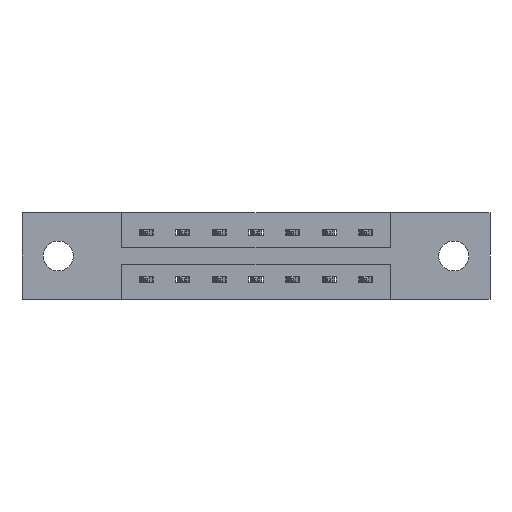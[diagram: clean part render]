
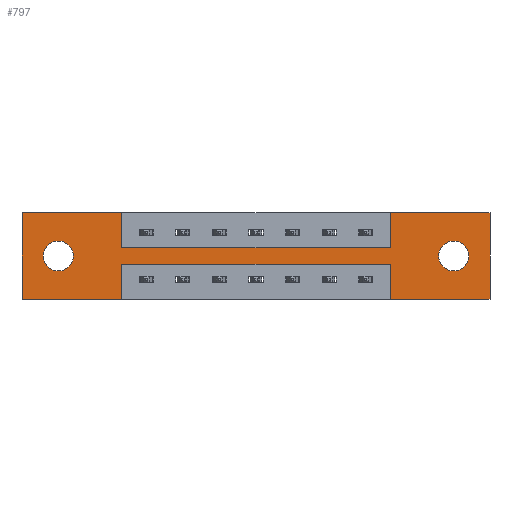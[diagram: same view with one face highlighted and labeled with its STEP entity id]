
A CAD part, front view. The second image highlights one B-rep face of the part: STEP entity #797.
In plain terms, the highlighted planar face has unit normal (0, -1, 0).
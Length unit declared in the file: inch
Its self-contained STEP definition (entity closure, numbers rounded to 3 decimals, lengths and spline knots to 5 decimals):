
#57 = VERTEX_POINT ( 'NONE', #1873 ) ;
#102 = VERTEX_POINT ( 'NONE', #5075 ) ;
#193 = DIRECTION ( 'NONE',  ( 0., 0., -1. ) ) ;
#246 = VERTEX_POINT ( 'NONE', #479 ) ;
#252 = LINE ( 'NONE', #4655, #4242 ) ;
#346 = VECTOR ( 'NONE', #427, 39.37008 ) ;
#351 = DIRECTION ( 'NONE',  ( 0., 1., 0. ) ) ;
#427 = DIRECTION ( 'NONE',  ( 0., 0., -1. ) ) ;
#438 = EDGE_CURVE ( 'NONE', #57, #654, #252, .T. ) ;
#441 = CARTESIAN_POINT ( 'NONE',  ( 1.573, 0., 0. ) ) ;
#479 = CARTESIAN_POINT ( 'NONE',  ( 0.425, 0., -0.37 ) ) ;
#485 = FACE_OUTER_BOUND ( 'NONE', #1655, .T. ) ;
#576 = CARTESIAN_POINT ( 'NONE',  ( 0., 0., -0.37 ) ) ;
#596 = CARTESIAN_POINT ( 'NONE',  ( 1.573, 0., -0.15 ) ) ;
#632 = CARTESIAN_POINT ( 'NONE',  ( 1.843, 0., -0.185 ) ) ;
#654 = VERTEX_POINT ( 'NONE', #596 ) ;
#797 = ADVANCED_FACE ( 'NONE', ( #4979, #7053, #485 ), #3371, .T. ) ;
#1040 = LINE ( 'NONE', #7191, #7038 ) ;
#1125 = VERTEX_POINT ( 'NONE', #5251 ) ;
#1134 = AXIS2_PLACEMENT_3D ( 'NONE', #632, #6412, #1499 ) ;
#1192 = VERTEX_POINT ( 'NONE', #7142 ) ;
#1312 = DIRECTION ( 'NONE',  ( 0., 0., 1. ) ) ;
#1349 = CARTESIAN_POINT ( 'NONE',  ( 0., 0., -0.37 ) ) ;
#1387 = EDGE_CURVE ( 'NONE', #5146, #7256, #3457, .T. ) ;
#1460 = VECTOR ( 'NONE', #3967, 39.37008 ) ;
#1499 = DIRECTION ( 'NONE',  ( 0., 0., -1. ) ) ;
#1594 = DIRECTION ( 'NONE',  ( 0., 0., 1. ) ) ;
#1655 = EDGE_LOOP ( 'NONE', ( #7145, #7356, #8476, #3352, #7436, #7718, #9291, #8265, #8059, #3949, #8338, #2180 ) ) ;
#1659 = CARTESIAN_POINT ( 'NONE',  ( 0., 0., 0. ) ) ;
#1700 = DIRECTION ( 'NONE',  ( 0., -1., 0. ) ) ;
#1873 = CARTESIAN_POINT ( 'NONE',  ( 0.425, 0., -0.15 ) ) ;
#2180 = ORIENTED_EDGE ( 'NONE', *, *, #7751, .F. ) ;
#2615 = LINE ( 'NONE', #4359, #6383 ) ;
#2652 = EDGE_CURVE ( 'NONE', #4081, #5425, #7710, .T. ) ;
#2749 = VERTEX_POINT ( 'NONE', #5734 ) ;
#2812 = DIRECTION ( 'NONE',  ( 0., 0., 1. ) ) ;
#2935 = AXIS2_PLACEMENT_3D ( 'NONE', #4027, #3998, #4519 ) ;
#2937 = EDGE_CURVE ( 'NONE', #1192, #1125, #3142, .T. ) ;
#2939 = CARTESIAN_POINT ( 'NONE',  ( 1.998, 0., 0. ) ) ;
#2958 = CARTESIAN_POINT ( 'NONE',  ( 1.843, 0., -0.249 ) ) ;
#2991 = AXIS2_PLACEMENT_3D ( 'NONE', #1349, #1700, #193 ) ;
#3142 = LINE ( 'NONE', #2939, #5064 ) ;
#3281 = DIRECTION ( 'NONE',  ( 1., 0., 0. ) ) ;
#3318 = CIRCLE ( 'NONE', #1134, 0.064 ) ;
#3352 = ORIENTED_EDGE ( 'NONE', *, *, #4785, .F. ) ;
#3371 = PLANE ( 'NONE',  #2991 ) ;
#3381 = DIRECTION ( 'NONE',  ( 0., 0., 1. ) ) ;
#3391 = CIRCLE ( 'NONE', #8374, 0.064 ) ;
#3427 = CARTESIAN_POINT ( 'NONE',  ( 1.843, 0., -0.121 ) ) ;
#3457 = CIRCLE ( 'NONE', #2935, 0.064 ) ;
#3515 = EDGE_CURVE ( 'NONE', #5425, #2749, #5433, .T. ) ;
#3530 = CARTESIAN_POINT ( 'NONE',  ( 0.155, 0., -0.185 ) ) ;
#3744 = LINE ( 'NONE', #9733, #1460 ) ;
#3860 = EDGE_CURVE ( 'NONE', #2749, #246, #2615, .T. ) ;
#3949 = ORIENTED_EDGE ( 'NONE', *, *, #9579, .F. ) ;
#3967 = DIRECTION ( 'NONE',  ( 1., 0., 0. ) ) ;
#3998 = DIRECTION ( 'NONE',  ( 0., 1., 0. ) ) ;
#4027 = CARTESIAN_POINT ( 'NONE',  ( 1.843, 0., -0.185 ) ) ;
#4081 = VERTEX_POINT ( 'NONE', #7683 ) ;
#4096 = DIRECTION ( 'NONE',  ( 0., 0., -1. ) ) ;
#4111 = VECTOR ( 'NONE', #3381, 39.37008 ) ;
#4159 = EDGE_CURVE ( 'NONE', #8902, #4447, #3391, .T. ) ;
#4242 = VECTOR ( 'NONE', #3281, 39.37008 ) ;
#4283 = DIRECTION ( 'NONE',  ( 0., 0., -1. ) ) ;
#4335 = VECTOR ( 'NONE', #1312, 39.37008 ) ;
#4345 = DIRECTION ( 'NONE',  ( 0., 0., 1. ) ) ;
#4359 = CARTESIAN_POINT ( 'NONE',  ( 0.425, 0., -0.37 ) ) ;
#4403 = VECTOR ( 'NONE', #5453, 39.37008 ) ;
#4447 = VERTEX_POINT ( 'NONE', #5831 ) ;
#4519 = DIRECTION ( 'NONE',  ( 0., 0., -1. ) ) ;
#4528 = ORIENTED_EDGE ( 'NONE', *, *, #1387, .T. ) ;
#4638 = LINE ( 'NONE', #576, #4403 ) ;
#4655 = CARTESIAN_POINT ( 'NONE',  ( 0.425, 0., -0.15 ) ) ;
#4785 = EDGE_CURVE ( 'NONE', #1125, #4081, #4638, .T. ) ;
#4979 = FACE_BOUND ( 'NONE', #6497, .T. ) ;
#5064 = VECTOR ( 'NONE', #4283, 39.37008 ) ;
#5075 = CARTESIAN_POINT ( 'NONE',  ( 0.425, 0., 0. ) ) ;
#5146 = VERTEX_POINT ( 'NONE', #2958 ) ;
#5251 = CARTESIAN_POINT ( 'NONE',  ( 1.998, 0., -0.37 ) ) ;
#5334 = AXIS2_PLACEMENT_3D ( 'NONE', #3530, #8789, #4345 ) ;
#5425 = VERTEX_POINT ( 'NONE', #6099 ) ;
#5433 = LINE ( 'NONE', #6477, #7234 ) ;
#5453 = DIRECTION ( 'NONE',  ( -1., 0., 0. ) ) ;
#5498 = CIRCLE ( 'NONE', #5334, 0.064 ) ;
#5620 = CARTESIAN_POINT ( 'NONE',  ( 0.155, 0., -0.185 ) ) ;
#5654 = DIRECTION ( 'NONE',  ( 1., 0., 0. ) ) ;
#5734 = CARTESIAN_POINT ( 'NONE',  ( 0.425, 0., -0.22 ) ) ;
#5831 = CARTESIAN_POINT ( 'NONE',  ( 0.155, 0., -0.121 ) ) ;
#5986 = VERTEX_POINT ( 'NONE', #6105 ) ;
#6099 = CARTESIAN_POINT ( 'NONE',  ( 1.573, 0., -0.22 ) ) ;
#6105 = CARTESIAN_POINT ( 'NONE',  ( 0., 0., 0. ) ) ;
#6177 = VECTOR ( 'NONE', #1594, 39.37008 ) ;
#6181 = LINE ( 'NONE', #441, #4335 ) ;
#6213 = CARTESIAN_POINT ( 'NONE',  ( 1.573, 0., -0.37 ) ) ;
#6383 = VECTOR ( 'NONE', #4096, 39.37008 ) ;
#6412 = DIRECTION ( 'NONE',  ( 0., 1., 0. ) ) ;
#6458 = ORIENTED_EDGE ( 'NONE', *, *, #7333, .T. ) ;
#6477 = CARTESIAN_POINT ( 'NONE',  ( 0.425, 0., -0.22 ) ) ;
#6497 = EDGE_LOOP ( 'NONE', ( #6967, #4528 ) ) ;
#6915 = LINE ( 'NONE', #9670, #346 ) ;
#6967 = ORIENTED_EDGE ( 'NONE', *, *, #9546, .T. ) ;
#7012 = EDGE_CURVE ( 'NONE', #9597, #1192, #3744, .T. ) ;
#7038 = VECTOR ( 'NONE', #5654, 39.37008 ) ;
#7046 = DIRECTION ( 'NONE',  ( -1., 0., 0. ) ) ;
#7053 = FACE_BOUND ( 'NONE', #8880, .T. ) ;
#7142 = CARTESIAN_POINT ( 'NONE',  ( 1.998, 0., 0. ) ) ;
#7145 = ORIENTED_EDGE ( 'NONE', *, *, #3860, .F. ) ;
#7191 = CARTESIAN_POINT ( 'NONE',  ( 0., 0., 0. ) ) ;
#7201 = CARTESIAN_POINT ( 'NONE',  ( 0., 0., -0.37 ) ) ;
#7215 = CARTESIAN_POINT ( 'NONE',  ( 1.573, 0., 0. ) ) ;
#7220 = EDGE_CURVE ( 'NONE', #8665, #5986, #9886, .T. ) ;
#7234 = VECTOR ( 'NONE', #7598, 39.37008 ) ;
#7256 = VERTEX_POINT ( 'NONE', #3427 ) ;
#7333 = EDGE_CURVE ( 'NONE', #4447, #8902, #5498, .T. ) ;
#7344 = ORIENTED_EDGE ( 'NONE', *, *, #4159, .T. ) ;
#7356 = ORIENTED_EDGE ( 'NONE', *, *, #3515, .F. ) ;
#7436 = ORIENTED_EDGE ( 'NONE', *, *, #2937, .F. ) ;
#7598 = DIRECTION ( 'NONE',  ( -1., 0., 0. ) ) ;
#7683 = CARTESIAN_POINT ( 'NONE',  ( 1.573, 0., -0.37 ) ) ;
#7710 = LINE ( 'NONE', #6213, #6177 ) ;
#7718 = ORIENTED_EDGE ( 'NONE', *, *, #7012, .F. ) ;
#7751 = EDGE_CURVE ( 'NONE', #246, #8665, #9250, .T. ) ;
#8059 = ORIENTED_EDGE ( 'NONE', *, *, #9356, .F. ) ;
#8101 = CARTESIAN_POINT ( 'NONE',  ( 0.155, 0., -0.249 ) ) ;
#8265 = ORIENTED_EDGE ( 'NONE', *, *, #438, .F. ) ;
#8338 = ORIENTED_EDGE ( 'NONE', *, *, #7220, .F. ) ;
#8374 = AXIS2_PLACEMENT_3D ( 'NONE', #5620, #351, #2812 ) ;
#8476 = ORIENTED_EDGE ( 'NONE', *, *, #2652, .F. ) ;
#8503 = EDGE_CURVE ( 'NONE', #654, #9597, #6181, .T. ) ;
#8665 = VERTEX_POINT ( 'NONE', #7201 ) ;
#8789 = DIRECTION ( 'NONE',  ( 0., 1., 0. ) ) ;
#8880 = EDGE_LOOP ( 'NONE', ( #6458, #7344 ) ) ;
#8902 = VERTEX_POINT ( 'NONE', #8101 ) ;
#9052 = VECTOR ( 'NONE', #7046, 39.37008 ) ;
#9250 = LINE ( 'NONE', #9689, #9052 ) ;
#9291 = ORIENTED_EDGE ( 'NONE', *, *, #8503, .F. ) ;
#9356 = EDGE_CURVE ( 'NONE', #102, #57, #6915, .T. ) ;
#9546 = EDGE_CURVE ( 'NONE', #7256, #5146, #3318, .T. ) ;
#9579 = EDGE_CURVE ( 'NONE', #5986, #102, #1040, .T. ) ;
#9597 = VERTEX_POINT ( 'NONE', #7215 ) ;
#9670 = CARTESIAN_POINT ( 'NONE',  ( 0.425, 0., 0. ) ) ;
#9689 = CARTESIAN_POINT ( 'NONE',  ( 0., 0., -0.37 ) ) ;
#9733 = CARTESIAN_POINT ( 'NONE',  ( 0., 0., 0. ) ) ;
#9886 = LINE ( 'NONE', #1659, #4111 ) ;
